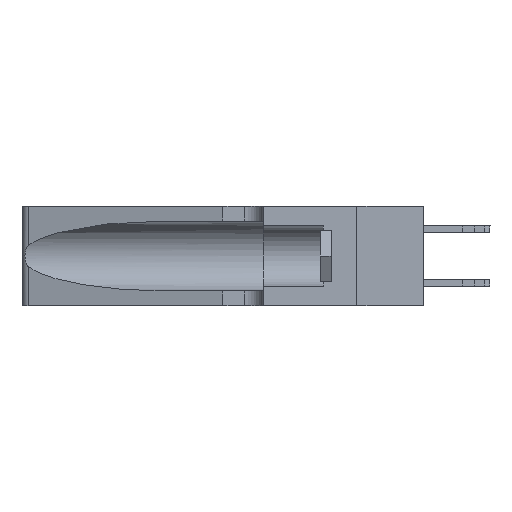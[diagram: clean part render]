
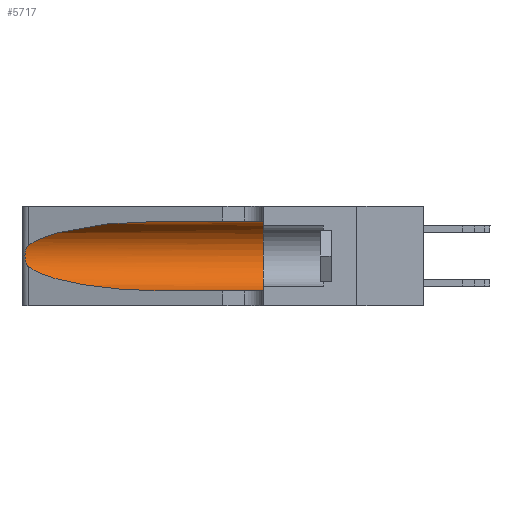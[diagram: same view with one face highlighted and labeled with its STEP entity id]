
A CAD part, left-side view. The second image highlights one B-rep face of the part: STEP entity #5717.
In plain terms, the highlighted cylindrical face has radius 3.308 mm (diameter 6.617 mm), a partial arc.
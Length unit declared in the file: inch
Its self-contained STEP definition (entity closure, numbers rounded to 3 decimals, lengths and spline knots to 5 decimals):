
#169 = DIRECTION ( 'NONE',  ( 0., 0., 1. ) ) ;
#1302 = CARTESIAN_POINT ( 'NONE',  ( 0.25487, 1.22718, 0.14631 ) ) ;
#1343 = ORIENTED_EDGE ( 'NONE', *, *, #19407, .T. ) ;
#1525 = VERTEX_POINT ( 'NONE', #21708 ) ;
#1696 = VERTEX_POINT ( 'NONE', #13770 ) ;
#1860 = DIRECTION ( 'NONE',  ( 0., -1., 0. ) ) ;
#2307 = ORIENTED_EDGE ( 'NONE', *, *, #16317, .T. ) ;
#2549 = CARTESIAN_POINT ( 'NONE',  ( 0.26075, 1.23896, 0.178 ) ) ;
#3020 = CARTESIAN_POINT ( 'NONE',  ( 0.1305, 0.72297, 0.05475 ) ) ;
#3501 = ORIENTED_EDGE ( 'NONE', *, *, #18651, .T. ) ;
#3745 = DIRECTION ( 'NONE',  ( 0., 1., 0. ) ) ;
#5717 = ADVANCED_FACE ( 'NONE', ( #21634 ), #15502, .F. ) ;
#5960 = CARTESIAN_POINT ( 'NONE',  ( 0.25789, 1.23486, 0.15765 ) ) ;
#6093 =( BOUNDED_CURVE ( )  B_SPLINE_CURVE ( 3, ( #11396, #6332, #6118, #19918 ),
 .UNSPECIFIED., .F., .T. ) 
 B_SPLINE_CURVE_WITH_KNOTS ( ( 4, 4 ),
 ( 1.5708, 2.84003 ),
 .UNSPECIFIED. ) 
 CURVE ( )  GEOMETRIC_REPRESENTATION_ITEM ( )  RATIONAL_B_SPLINE_CURVE ( ( 1., 0.87, 0.87, 1. ) ) 
 REPRESENTATION_ITEM ( '' )  );
#6118 = CARTESIAN_POINT ( 'NONE',  ( 0.2373, 1.15595, 0.28018 ) ) ;
#6332 = CARTESIAN_POINT ( 'NONE',  ( 0.18966, 0.96281, 0.31525 ) ) ;
#7006 = CARTESIAN_POINT ( 'NONE',  ( 0.1305, 0.72297, 0.05475 ) ) ;
#7175 = ORIENTED_EDGE ( 'NONE', *, *, #15506, .F. ) ;
#7462 = CARTESIAN_POINT ( 'NONE',  ( 0.1305, 0.72297, 0.31525 ) ) ;
#7600 = CARTESIAN_POINT ( 'NONE',  ( 0.25854, 1.2359, 0.20912 ) ) ;
#7770 = VERTEX_POINT ( 'NONE', #7006 ) ;
#7894 = CARTESIAN_POINT ( 'NONE',  ( 0.25639, 1.23186, 0.15144 ) ) ;
#8026 = CARTESIAN_POINT ( 'NONE',  ( 0.25487, 1.22718, 0.14631 ) ) ;
#8161 = LINE ( 'NONE', #19428, #9240 ) ;
#8757 = CARTESIAN_POINT ( 'NONE',  ( 0.1305, 0.35, 0.31525 ) ) ;
#9125 = EDGE_LOOP ( 'NONE', ( #2307, #18774, #3501, #1343, #20111, #7175 ) ) ;
#9240 = VECTOR ( 'NONE', #17570, 39.37008 ) ;
#9310 = CARTESIAN_POINT ( 'NONE',  ( 0.26018, 1.23835, 0.19895 ) ) ;
#9330 = LINE ( 'NONE', #13436, #15478 ) ;
#9365 =( BOUNDED_CURVE ( )  B_SPLINE_CURVE ( 3, ( #1302, #13320, #14963, #3020 ),
 .UNSPECIFIED., .F., .T. ) 
 B_SPLINE_CURVE_WITH_KNOTS ( ( 4, 4 ),
 ( 3.44316, 4.71239 ),
 .UNSPECIFIED. ) 
 CURVE ( )  GEOMETRIC_REPRESENTATION_ITEM ( )  RATIONAL_B_SPLINE_CURVE ( ( 1., 0.87, 0.87, 1. ) ) 
 REPRESENTATION_ITEM ( '' )  );
#9376 = CARTESIAN_POINT ( 'NONE',  ( 0.25856, 1.23593, 0.16098 ) ) ;
#9756 = DIRECTION ( 'NONE',  ( 0., -1., 0. ) ) ;
#9815 = CIRCLE ( 'NONE', #18328, 0.13025 ) ;
#10343 = B_SPLINE_CURVE_WITH_KNOTS ( 'NONE', 3,
 ( #19468, #11161, #10949, #14591, #7600, #9310, #12738, #2549, #14439, #9376, #5960, #7894, #14883, #8026 ),
 .UNSPECIFIED., .F., .F.,
 ( 4, 2, 2, 2, 2, 2, 4 ),
 ( 0., 0.00027, 0.00053, 0.00107, 0.0016, 0.00187, 0.00214 ),
 .UNSPECIFIED. ) ;
#10949 = CARTESIAN_POINT ( 'NONE',  ( 0.25639, 1.23184, 0.21858 ) ) ;
#11161 = CARTESIAN_POINT ( 'NONE',  ( 0.25555, 1.22994, 0.2215 ) ) ;
#11307 = CARTESIAN_POINT ( 'NONE',  ( 0.1305, 1.61858, 0.185 ) ) ;
#11396 = CARTESIAN_POINT ( 'NONE',  ( 0.1305, 0.72297, 0.31525 ) ) ;
#11507 = CARTESIAN_POINT ( 'NONE',  ( 0.25487, 1.22718, 0.22369 ) ) ;
#12738 = CARTESIAN_POINT ( 'NONE',  ( 0.26075, 1.23896, 0.19203 ) ) ;
#12957 = DIRECTION ( 'NONE',  ( 0., 0., -1. ) ) ;
#13320 = CARTESIAN_POINT ( 'NONE',  ( 0.2373, 1.15595, 0.08982 ) ) ;
#13436 = CARTESIAN_POINT ( 'NONE',  ( 0.1305, 1.61858, 0.05475 ) ) ;
#13672 = CARTESIAN_POINT ( 'NONE',  ( 0.1305, 0.35, 0.185 ) ) ;
#13770 = CARTESIAN_POINT ( 'NONE',  ( 0.1305, 0.35, 0.05475 ) ) ;
#14439 = CARTESIAN_POINT ( 'NONE',  ( 0.26017, 1.23833, 0.17102 ) ) ;
#14591 = CARTESIAN_POINT ( 'NONE',  ( 0.25787, 1.23484, 0.2124 ) ) ;
#14883 = CARTESIAN_POINT ( 'NONE',  ( 0.25555, 1.22993, 0.14849 ) ) ;
#14963 = CARTESIAN_POINT ( 'NONE',  ( 0.18966, 0.96281, 0.05475 ) ) ;
#15478 = VECTOR ( 'NONE', #1860, 39.37008 ) ;
#15502 = CYLINDRICAL_SURFACE ( 'NONE', #17864, 0.13025 ) ;
#15506 = EDGE_CURVE ( 'NONE', #18287, #19602, #8161, .T. ) ;
#16317 = EDGE_CURVE ( 'NONE', #18287, #21244, #6093, .T. ) ;
#17570 = DIRECTION ( 'NONE',  ( 0., -1., 0. ) ) ;
#17864 = AXIS2_PLACEMENT_3D ( 'NONE', #11307, #9756, #12957 ) ;
#18287 = VERTEX_POINT ( 'NONE', #7462 ) ;
#18328 = AXIS2_PLACEMENT_3D ( 'NONE', #13672, #3745, #169 ) ;
#18651 = EDGE_CURVE ( 'NONE', #1525, #7770, #9365, .T. ) ;
#18774 = ORIENTED_EDGE ( 'NONE', *, *, #20654, .T. ) ;
#19407 = EDGE_CURVE ( 'NONE', #7770, #1696, #9330, .T. ) ;
#19428 = CARTESIAN_POINT ( 'NONE',  ( 0.1305, 1.61858, 0.31525 ) ) ;
#19468 = CARTESIAN_POINT ( 'NONE',  ( 0.25487, 1.22718, 0.22369 ) ) ;
#19602 = VERTEX_POINT ( 'NONE', #8757 ) ;
#19918 = CARTESIAN_POINT ( 'NONE',  ( 0.25487, 1.22718, 0.22369 ) ) ;
#20111 = ORIENTED_EDGE ( 'NONE', *, *, #20964, .F. ) ;
#20654 = EDGE_CURVE ( 'NONE', #21244, #1525, #10343, .T. ) ;
#20964 = EDGE_CURVE ( 'NONE', #19602, #1696, #9815, .T. ) ;
#21244 = VERTEX_POINT ( 'NONE', #11507 ) ;
#21634 = FACE_OUTER_BOUND ( 'NONE', #9125, .T. ) ;
#21708 = CARTESIAN_POINT ( 'NONE',  ( 0.25487, 1.22718, 0.14631 ) ) ;
